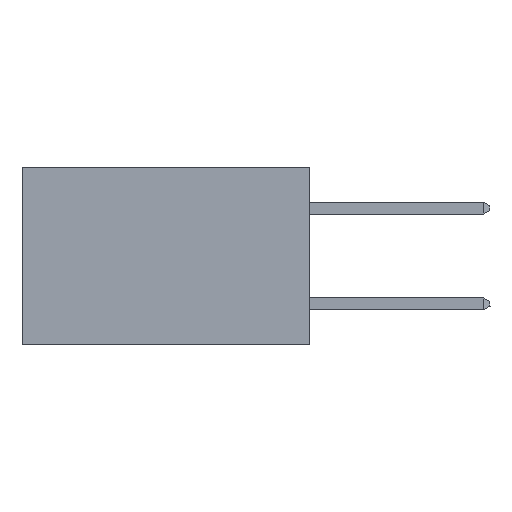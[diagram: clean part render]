
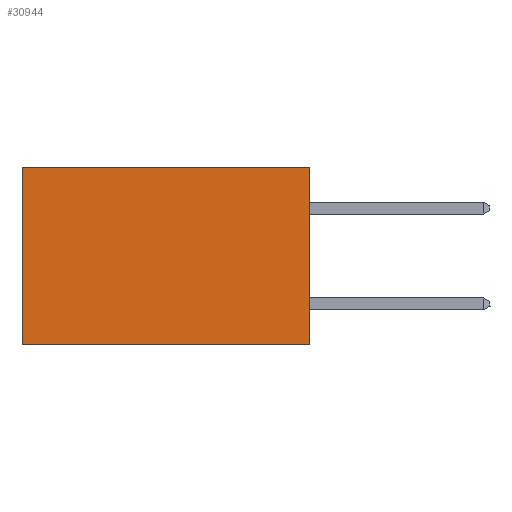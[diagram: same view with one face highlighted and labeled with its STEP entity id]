
A CAD part, left-side view. The second image highlights one B-rep face of the part: STEP entity #30944.
In plain terms, the highlighted planar face has unit normal (-1, 0, 0).
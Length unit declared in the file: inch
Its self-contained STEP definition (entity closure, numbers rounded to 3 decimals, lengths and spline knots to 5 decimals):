
#298 = LINE ( 'NONE', #15034, #17004 ) ;
#623 = CARTESIAN_POINT ( 'NONE',  ( 0.2875, 0., -0.37 ) ) ;
#715 = CARTESIAN_POINT ( 'NONE',  ( 0.2875, 0., 0. ) ) ;
#3021 = DIRECTION ( 'NONE',  ( 0., 0., -1. ) ) ;
#4256 = CARTESIAN_POINT ( 'NONE',  ( 0.2875, 0.6, -0.37 ) ) ;
#4731 = VERTEX_POINT ( 'NONE', #623 ) ;
#5274 = LINE ( 'NONE', #32179, #27404 ) ;
#5458 = VECTOR ( 'NONE', #19662, 39.37008 ) ;
#8124 = DIRECTION ( 'NONE',  ( 1., 0., 0. ) ) ;
#8960 = VERTEX_POINT ( 'NONE', #30736 ) ;
#9486 = FACE_OUTER_BOUND ( 'NONE', #18678, .T. ) ;
#12267 = EDGE_CURVE ( 'NONE', #38948, #8960, #37788, .T. ) ;
#12832 = VERTEX_POINT ( 'NONE', #4256 ) ;
#13400 = ORIENTED_EDGE ( 'NONE', *, *, #19689, .F. ) ;
#14306 = PLANE ( 'NONE',  #19230 ) ;
#15034 = CARTESIAN_POINT ( 'NONE',  ( 0.2875, 0., 0. ) ) ;
#17004 = VECTOR ( 'NONE', #24563, 39.37008 ) ;
#18678 = EDGE_LOOP ( 'NONE', ( #23479, #32643, #13400, #22533 ) ) ;
#19230 = AXIS2_PLACEMENT_3D ( 'NONE', #26988, #8124, #30121 ) ;
#19662 = DIRECTION ( 'NONE',  ( 0., 1., 0. ) ) ;
#19689 = EDGE_CURVE ( 'NONE', #38948, #4731, #298, .T. ) ;
#22533 = ORIENTED_EDGE ( 'NONE', *, *, #12267, .T. ) ;
#23479 = ORIENTED_EDGE ( 'NONE', *, *, #29433, .T. ) ;
#24322 = VECTOR ( 'NONE', #3021, 39.37008 ) ;
#24563 = DIRECTION ( 'NONE',  ( 0., 0., -1. ) ) ;
#25307 = LINE ( 'NONE', #28169, #24322 ) ;
#26988 = CARTESIAN_POINT ( 'NONE',  ( 0.2875, 0., 0. ) ) ;
#27404 = VECTOR ( 'NONE', #35295, 39.37008 ) ;
#27929 = CARTESIAN_POINT ( 'NONE',  ( 0.2875, 0., 0. ) ) ;
#28169 = CARTESIAN_POINT ( 'NONE',  ( 0.2875, 0.6, 0. ) ) ;
#29433 = EDGE_CURVE ( 'NONE', #8960, #12832, #25307, .T. ) ;
#30121 = DIRECTION ( 'NONE',  ( 0., 0., -1. ) ) ;
#30736 = CARTESIAN_POINT ( 'NONE',  ( 0.2875, 0.6, 0. ) ) ;
#30944 = ADVANCED_FACE ( 'NONE', ( #9486 ), #14306, .F. ) ;
#32179 = CARTESIAN_POINT ( 'NONE',  ( 0.2875, 0., -0.37 ) ) ;
#32643 = ORIENTED_EDGE ( 'NONE', *, *, #38543, .F. ) ;
#35295 = DIRECTION ( 'NONE',  ( 0., 1., 0. ) ) ;
#37788 = LINE ( 'NONE', #715, #5458 ) ;
#38543 = EDGE_CURVE ( 'NONE', #4731, #12832, #5274, .T. ) ;
#38948 = VERTEX_POINT ( 'NONE', #27929 ) ;
